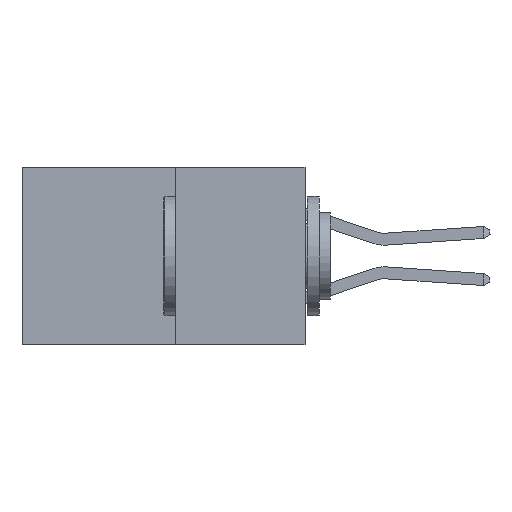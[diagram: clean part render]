
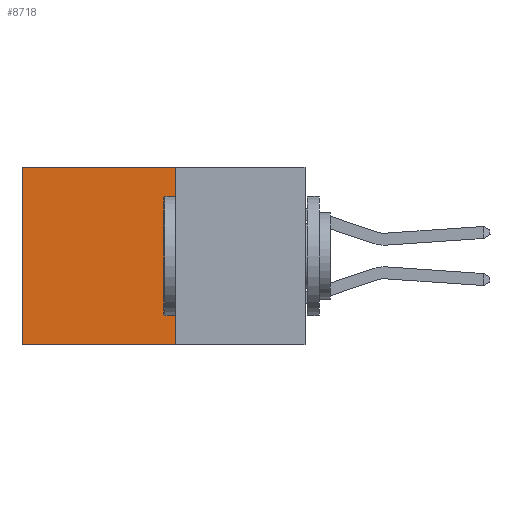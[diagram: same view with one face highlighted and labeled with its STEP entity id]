
A CAD part, left-side view. The second image highlights one B-rep face of the part: STEP entity #8718.
In plain terms, the highlighted planar face has unit normal (-1, 0, 0).
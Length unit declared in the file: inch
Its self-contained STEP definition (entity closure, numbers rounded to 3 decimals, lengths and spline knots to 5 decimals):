
#66 = VERTEX_POINT ( 'NONE', #17266 ) ;
#821 = CARTESIAN_POINT ( 'NONE',  ( 0.277, 0.59, 0. ) ) ;
#1523 = DIRECTION ( 'NONE',  ( 0., 1., 0. ) ) ;
#1562 = PLANE ( 'NONE',  #12894 ) ;
#2641 = VERTEX_POINT ( 'NONE', #9351 ) ;
#3668 = DIRECTION ( 'NONE',  ( 0., 0., -1. ) ) ;
#3774 = CARTESIAN_POINT ( 'NONE',  ( 0.277, 0.27, -0.37 ) ) ;
#4154 = VECTOR ( 'NONE', #1523, 39.37008 ) ;
#4537 = EDGE_CURVE ( 'NONE', #66, #14923, #10236, .T. ) ;
#4613 = LINE ( 'NONE', #3774, #4154 ) ;
#5059 = EDGE_LOOP ( 'NONE', ( #15381, #13277, #11667, #13515 ) ) ;
#5198 = VECTOR ( 'NONE', #7001, 39.37008 ) ;
#5982 = VECTOR ( 'NONE', #12528, 39.37008 ) ;
#7001 = DIRECTION ( 'NONE',  ( 0., 0., -1. ) ) ;
#7617 = DIRECTION ( 'NONE',  ( 1., 0., 0. ) ) ;
#8038 = CARTESIAN_POINT ( 'NONE',  ( 0.277, 0.27, -0.37 ) ) ;
#8248 = EDGE_CURVE ( 'NONE', #2641, #13252, #4613, .T. ) ;
#8718 = ADVANCED_FACE ( 'NONE', ( #11688 ), #1562, .F. ) ;
#9351 = CARTESIAN_POINT ( 'NONE',  ( 0.277, 0.27, -0.37 ) ) ;
#9751 = VECTOR ( 'NONE', #19340, 39.37008 ) ;
#10023 = LINE ( 'NONE', #8038, #5982 ) ;
#10236 = LINE ( 'NONE', #11380, #9751 ) ;
#10533 = EDGE_CURVE ( 'NONE', #66, #2641, #10023, .T. ) ;
#10715 = CARTESIAN_POINT ( 'NONE',  ( 0.277, 0.27, -0.37 ) ) ;
#11380 = CARTESIAN_POINT ( 'NONE',  ( 0.277, 0.27, 0. ) ) ;
#11667 = ORIENTED_EDGE ( 'NONE', *, *, #10533, .F. ) ;
#11688 = FACE_OUTER_BOUND ( 'NONE', #5059, .T. ) ;
#12528 = DIRECTION ( 'NONE',  ( 0., 0., -1. ) ) ;
#12894 = AXIS2_PLACEMENT_3D ( 'NONE', #10715, #7617, #3668 ) ;
#12948 = CARTESIAN_POINT ( 'NONE',  ( 0.277, 0.59, -0.37 ) ) ;
#13252 = VERTEX_POINT ( 'NONE', #16397 ) ;
#13277 = ORIENTED_EDGE ( 'NONE', *, *, #8248, .F. ) ;
#13515 = ORIENTED_EDGE ( 'NONE', *, *, #4537, .T. ) ;
#14923 = VERTEX_POINT ( 'NONE', #821 ) ;
#15381 = ORIENTED_EDGE ( 'NONE', *, *, #18449, .T. ) ;
#16397 = CARTESIAN_POINT ( 'NONE',  ( 0.277, 0.59, -0.37 ) ) ;
#17242 = LINE ( 'NONE', #12948, #5198 ) ;
#17266 = CARTESIAN_POINT ( 'NONE',  ( 0.277, 0.27, 0. ) ) ;
#18449 = EDGE_CURVE ( 'NONE', #14923, #13252, #17242, .T. ) ;
#19340 = DIRECTION ( 'NONE',  ( 0., 1., 0. ) ) ;
